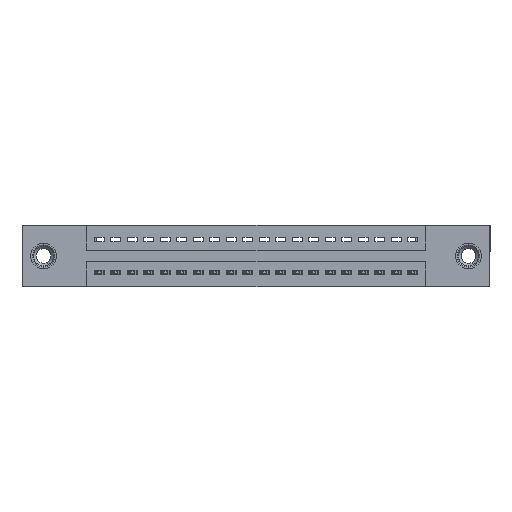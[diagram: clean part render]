
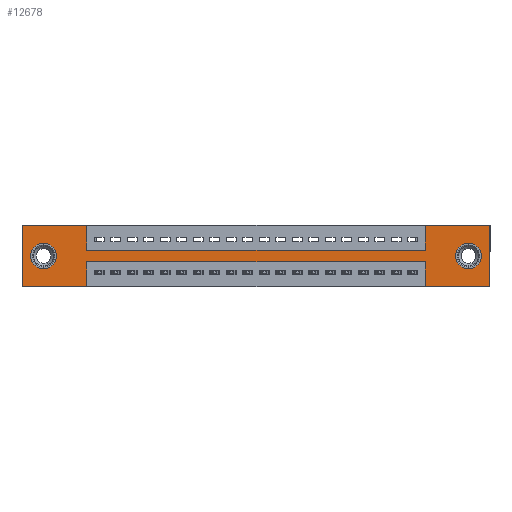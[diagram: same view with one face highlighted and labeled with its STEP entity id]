
A CAD part, front view. The second image highlights one B-rep face of the part: STEP entity #12678.
In plain terms, the highlighted planar face has unit normal (0, -1, 0).
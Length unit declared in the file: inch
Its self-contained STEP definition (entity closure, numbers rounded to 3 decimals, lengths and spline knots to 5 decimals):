
#91 = EDGE_CURVE ( 'NONE', #15249, #921, #9933, .T. ) ;
#256 = DIRECTION ( 'NONE',  ( -1., 0., 0. ) ) ;
#591 = VERTEX_POINT ( 'NONE', #18504 ) ;
#709 = VECTOR ( 'NONE', #256, 39.37008 ) ;
#788 = DIRECTION ( 'NONE',  ( 1., 0., 0. ) ) ;
#822 = VERTEX_POINT ( 'NONE', #2312 ) ;
#921 = VERTEX_POINT ( 'NONE', #4629 ) ;
#1195 = VECTOR ( 'NONE', #14150, 39.37008 ) ;
#1301 = VERTEX_POINT ( 'NONE', #10469 ) ;
#1512 = CARTESIAN_POINT ( 'NONE',  ( 0., 0., 0. ) ) ;
#1897 = LINE ( 'NONE', #8177, #12568 ) ;
#1985 = VERTEX_POINT ( 'NONE', #5441 ) ;
#2151 = CARTESIAN_POINT ( 'NONE',  ( 2.4425, 0., -0.37 ) ) ;
#2173 = CARTESIAN_POINT ( 'NONE',  ( 2.4425, 0., -0.37 ) ) ;
#2240 = AXIS2_PLACEMENT_3D ( 'NONE', #16487, #19632, #8699 ) ;
#2312 = CARTESIAN_POINT ( 'NONE',  ( 0.3925, 0., -0.22 ) ) ;
#2349 = CARTESIAN_POINT ( 'NONE',  ( 2.835, 0., 0. ) ) ;
#2746 = EDGE_CURVE ( 'NONE', #591, #11766, #13377, .T. ) ;
#2916 = CARTESIAN_POINT ( 'NONE',  ( 0., 0., -0.37 ) ) ;
#2997 = DIRECTION ( 'NONE',  ( 0., 0., 1. ) ) ;
#3074 = DIRECTION ( 'NONE',  ( 0., 0., 1. ) ) ;
#3324 = EDGE_CURVE ( 'NONE', #11360, #1985, #17994, .T. ) ;
#3856 = EDGE_CURVE ( 'NONE', #12506, #11360, #9464, .T. ) ;
#4061 = VERTEX_POINT ( 'NONE', #16735 ) ;
#4328 = VERTEX_POINT ( 'NONE', #12511 ) ;
#4340 = DIRECTION ( 'NONE',  ( -1., 0., 0. ) ) ;
#4507 = VECTOR ( 'NONE', #4340, 39.37008 ) ;
#4519 = CARTESIAN_POINT ( 'NONE',  ( 0.3925, 0., 0. ) ) ;
#4629 = CARTESIAN_POINT ( 'NONE',  ( 0., 0., -0.37 ) ) ;
#4705 = FACE_BOUND ( 'NONE', #17465, .T. ) ;
#5441 = CARTESIAN_POINT ( 'NONE',  ( 2.835, 0., -0.37 ) ) ;
#5567 = DIRECTION ( 'NONE',  ( 0., 0., 1. ) ) ;
#5762 = CARTESIAN_POINT ( 'NONE',  ( 0.3925, 0., -0.22 ) ) ;
#5805 = EDGE_CURVE ( 'NONE', #1985, #17625, #9114, .T. ) ;
#5920 = FACE_OUTER_BOUND ( 'NONE', #12816, .T. ) ;
#6115 = EDGE_CURVE ( 'NONE', #14342, #1301, #17906, .T. ) ;
#6496 = CARTESIAN_POINT ( 'NONE',  ( 2.4425, 0., 0. ) ) ;
#6698 = DIRECTION ( 'NONE',  ( 0., 0., -1. ) ) ;
#6700 = VECTOR ( 'NONE', #18778, 39.37008 ) ;
#6770 = ORIENTED_EDGE ( 'NONE', *, *, #11764, .F. ) ;
#6889 = VECTOR ( 'NONE', #18222, 39.37008 ) ;
#6905 = EDGE_LOOP ( 'NONE', ( #18678, #9313 ) ) ;
#7123 = CARTESIAN_POINT ( 'NONE',  ( 0.3925, 0., -0.15 ) ) ;
#7465 = EDGE_CURVE ( 'NONE', #9163, #20112, #16125, .T. ) ;
#7749 = ORIENTED_EDGE ( 'NONE', *, *, #7465, .F. ) ;
#7980 = CARTESIAN_POINT ( 'NONE',  ( 0.3925, 0., -0.15 ) ) ;
#8173 = ORIENTED_EDGE ( 'NONE', *, *, #9803, .F. ) ;
#8177 = CARTESIAN_POINT ( 'NONE',  ( 0.3925, 0., -0.37 ) ) ;
#8181 = CARTESIAN_POINT ( 'NONE',  ( 0., 0., -0.37 ) ) ;
#8236 = ORIENTED_EDGE ( 'NONE', *, *, #16015, .T. ) ;
#8314 = CARTESIAN_POINT ( 'NONE',  ( 0.13, 0., -0.263 ) ) ;
#8699 = DIRECTION ( 'NONE',  ( 0., 0., 1. ) ) ;
#9114 = LINE ( 'NONE', #2916, #4507 ) ;
#9163 = VERTEX_POINT ( 'NONE', #12709 ) ;
#9207 = AXIS2_PLACEMENT_3D ( 'NONE', #8181, #19326, #14461 ) ;
#9313 = ORIENTED_EDGE ( 'NONE', *, *, #19223, .T. ) ;
#9464 = LINE ( 'NONE', #14909, #1195 ) ;
#9598 = ORIENTED_EDGE ( 'NONE', *, *, #6115, .F. ) ;
#9631 = VECTOR ( 'NONE', #3074, 39.37008 ) ;
#9760 = VECTOR ( 'NONE', #2997, 39.37008 ) ;
#9803 = EDGE_CURVE ( 'NONE', #822, #15249, #1897, .T. ) ;
#9933 = LINE ( 'NONE', #18934, #709 ) ;
#10165 = VECTOR ( 'NONE', #10504, 39.37008 ) ;
#10318 = ORIENTED_EDGE ( 'NONE', *, *, #12829, .F. ) ;
#10469 = CARTESIAN_POINT ( 'NONE',  ( 2.4425, 0., -0.15 ) ) ;
#10504 = DIRECTION ( 'NONE',  ( 0., 0., -1. ) ) ;
#10835 = LINE ( 'NONE', #2173, #14537 ) ;
#11248 = DIRECTION ( 'NONE',  ( 0., 1., 0. ) ) ;
#11263 = CARTESIAN_POINT ( 'NONE',  ( 2.705, 0., -0.185 ) ) ;
#11360 = VERTEX_POINT ( 'NONE', #2349 ) ;
#11472 = LINE ( 'NONE', #5762, #6889 ) ;
#11564 = CARTESIAN_POINT ( 'NONE',  ( 0., 0., 0. ) ) ;
#11764 = EDGE_CURVE ( 'NONE', #20112, #14342, #13007, .T. ) ;
#11766 = VERTEX_POINT ( 'NONE', #13907 ) ;
#11996 = CARTESIAN_POINT ( 'NONE',  ( 2.835, 0., 0. ) ) ;
#12314 = DIRECTION ( 'NONE',  ( 0., 0., -1. ) ) ;
#12506 = VERTEX_POINT ( 'NONE', #6496 ) ;
#12511 = CARTESIAN_POINT ( 'NONE',  ( 2.4425, 0., -0.22 ) ) ;
#12568 = VECTOR ( 'NONE', #6698, 39.37008 ) ;
#12665 = LINE ( 'NONE', #1512, #9631 ) ;
#12678 = ADVANCED_FACE ( 'NONE', ( #13445, #4705, #5920 ), #12766, .T. ) ;
#12709 = CARTESIAN_POINT ( 'NONE',  ( 0., 0., 0. ) ) ;
#12766 = PLANE ( 'NONE',  #9207 ) ;
#12816 = EDGE_LOOP ( 'NONE', ( #8173, #10318, #14681, #13809, #14172, #13492, #17857, #9598, #6770, #7749, #16461, #16003 ) ) ;
#12829 = EDGE_CURVE ( 'NONE', #4328, #822, #11472, .T. ) ;
#13007 = LINE ( 'NONE', #4519, #14493 ) ;
#13131 = ORIENTED_EDGE ( 'NONE', *, *, #16156, .T. ) ;
#13312 = EDGE_CURVE ( 'NONE', #921, #9163, #12665, .T. ) ;
#13377 = CIRCLE ( 'NONE', #19909, 0.078 ) ;
#13445 = FACE_BOUND ( 'NONE', #6905, .T. ) ;
#13492 = ORIENTED_EDGE ( 'NONE', *, *, #3856, .F. ) ;
#13627 = CIRCLE ( 'NONE', #18191, 0.078 ) ;
#13809 = ORIENTED_EDGE ( 'NONE', *, *, #5805, .F. ) ;
#13887 = CARTESIAN_POINT ( 'NONE',  ( 0.13, 0., -0.185 ) ) ;
#13907 = CARTESIAN_POINT ( 'NONE',  ( 2.705, 0., -0.263 ) ) ;
#13942 = CARTESIAN_POINT ( 'NONE',  ( 2.4425, 0., 0. ) ) ;
#14150 = DIRECTION ( 'NONE',  ( 1., 0., 0. ) ) ;
#14172 = ORIENTED_EDGE ( 'NONE', *, *, #3324, .F. ) ;
#14224 = DIRECTION ( 'NONE',  ( 0., 0., -1. ) ) ;
#14342 = VERTEX_POINT ( 'NONE', #7123 ) ;
#14461 = DIRECTION ( 'NONE',  ( 0., 0., -1. ) ) ;
#14493 = VECTOR ( 'NONE', #12314, 39.37008 ) ;
#14537 = VECTOR ( 'NONE', #5567, 39.37008 ) ;
#14667 = CARTESIAN_POINT ( 'NONE',  ( 0.3925, 0., 0. ) ) ;
#14681 = ORIENTED_EDGE ( 'NONE', *, *, #15464, .F. ) ;
#14909 = CARTESIAN_POINT ( 'NONE',  ( 0., 0., 0. ) ) ;
#14985 = CIRCLE ( 'NONE', #16089, 0.078 ) ;
#15249 = VERTEX_POINT ( 'NONE', #15635 ) ;
#15464 = EDGE_CURVE ( 'NONE', #17625, #4328, #10835, .T. ) ;
#15635 = CARTESIAN_POINT ( 'NONE',  ( 0.3925, 0., -0.37 ) ) ;
#15975 = CIRCLE ( 'NONE', #2240, 0.078 ) ;
#16003 = ORIENTED_EDGE ( 'NONE', *, *, #91, .F. ) ;
#16015 = EDGE_CURVE ( 'NONE', #17242, #4061, #15975, .T. ) ;
#16089 = AXIS2_PLACEMENT_3D ( 'NONE', #13887, #18550, #18616 ) ;
#16125 = LINE ( 'NONE', #11564, #16596 ) ;
#16156 = EDGE_CURVE ( 'NONE', #4061, #17242, #14985, .T. ) ;
#16461 = ORIENTED_EDGE ( 'NONE', *, *, #13312, .F. ) ;
#16487 = CARTESIAN_POINT ( 'NONE',  ( 0.13, 0., -0.185 ) ) ;
#16596 = VECTOR ( 'NONE', #788, 39.37008 ) ;
#16735 = CARTESIAN_POINT ( 'NONE',  ( 0.13, 0., -0.107 ) ) ;
#17242 = VERTEX_POINT ( 'NONE', #8314 ) ;
#17442 = DIRECTION ( 'NONE',  ( 0., 0., -1. ) ) ;
#17465 = EDGE_LOOP ( 'NONE', ( #13131, #8236 ) ) ;
#17581 = DIRECTION ( 'NONE',  ( 0., 1., 0. ) ) ;
#17625 = VERTEX_POINT ( 'NONE', #2151 ) ;
#17857 = ORIENTED_EDGE ( 'NONE', *, *, #19134, .F. ) ;
#17906 = LINE ( 'NONE', #7980, #6700 ) ;
#17994 = LINE ( 'NONE', #11996, #10165 ) ;
#18066 = LINE ( 'NONE', #13942, #9760 ) ;
#18191 = AXIS2_PLACEMENT_3D ( 'NONE', #18816, #11248, #14224 ) ;
#18222 = DIRECTION ( 'NONE',  ( -1., 0., 0. ) ) ;
#18504 = CARTESIAN_POINT ( 'NONE',  ( 2.705, 0., -0.107 ) ) ;
#18550 = DIRECTION ( 'NONE',  ( 0., 1., 0. ) ) ;
#18616 = DIRECTION ( 'NONE',  ( 0., 0., 1. ) ) ;
#18678 = ORIENTED_EDGE ( 'NONE', *, *, #2746, .T. ) ;
#18778 = DIRECTION ( 'NONE',  ( 1., 0., 0. ) ) ;
#18816 = CARTESIAN_POINT ( 'NONE',  ( 2.705, 0., -0.185 ) ) ;
#18934 = CARTESIAN_POINT ( 'NONE',  ( 0., 0., -0.37 ) ) ;
#19134 = EDGE_CURVE ( 'NONE', #1301, #12506, #18066, .T. ) ;
#19223 = EDGE_CURVE ( 'NONE', #11766, #591, #13627, .T. ) ;
#19326 = DIRECTION ( 'NONE',  ( 0., -1., 0. ) ) ;
#19632 = DIRECTION ( 'NONE',  ( 0., 1., 0. ) ) ;
#19909 = AXIS2_PLACEMENT_3D ( 'NONE', #11263, #17581, #17442 ) ;
#20112 = VERTEX_POINT ( 'NONE', #14667 ) ;
